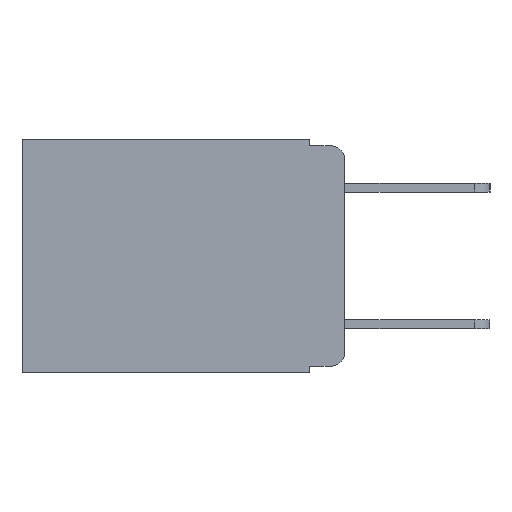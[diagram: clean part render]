
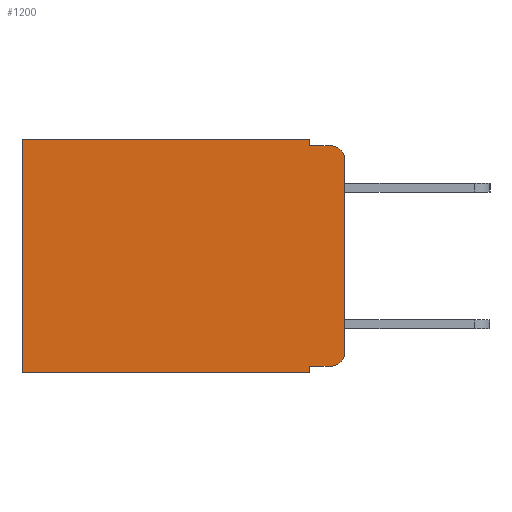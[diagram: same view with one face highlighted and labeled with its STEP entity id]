
A CAD part, left-side view. The second image highlights one B-rep face of the part: STEP entity #1200.
In plain terms, the highlighted planar face has unit normal (-1, 0, 0).
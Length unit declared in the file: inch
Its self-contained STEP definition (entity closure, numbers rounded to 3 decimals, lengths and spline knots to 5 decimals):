
#104 = DIRECTION ( 'NONE',  ( 0., 0., -1. ) ) ;
#127 = DIRECTION ( 'NONE',  ( -1., 0., 0. ) ) ;
#390 = LINE ( 'NONE', #4589, #6606 ) ;
#402 = DIRECTION ( 'NONE',  ( 1., 0., 0. ) ) ;
#555 = ORIENTED_EDGE ( 'NONE', *, *, #3717, .F. ) ;
#615 = VECTOR ( 'NONE', #10559, 39.37008 ) ;
#712 = VERTEX_POINT ( 'NONE', #10216 ) ;
#1023 = ORIENTED_EDGE ( 'NONE', *, *, #2513, .T. ) ;
#1200 = ADVANCED_FACE ( 'NONE', ( #3035 ), #11545, .F. ) ;
#1435 = ORIENTED_EDGE ( 'NONE', *, *, #3086, .F. ) ;
#1583 = CARTESIAN_POINT ( 'NONE',  ( 0.298, 0.02, -0.03 ) ) ;
#2192 = EDGE_CURVE ( 'NONE', #712, #9393, #390, .T. ) ;
#2199 = ORIENTED_EDGE ( 'NONE', *, *, #2450, .F. ) ;
#2424 = EDGE_CURVE ( 'NONE', #5941, #10983, #8377, .T. ) ;
#2448 = EDGE_CURVE ( 'NONE', #5403, #5941, #5868, .T. ) ;
#2450 = EDGE_CURVE ( 'NONE', #5403, #6132, #5561, .T. ) ;
#2513 = EDGE_CURVE ( 'NONE', #9393, #5995, #11016, .T. ) ;
#2515 = CARTESIAN_POINT ( 'NONE',  ( 0.298, 0.051, -0.333 ) ) ;
#2554 = AXIS2_PLACEMENT_3D ( 'NONE', #7008, #8761, #6050 ) ;
#2683 = ORIENTED_EDGE ( 'NONE', *, *, #3149, .F. ) ;
#2730 = DIRECTION ( 'NONE',  ( 0., 0., -1. ) ) ;
#3035 = FACE_OUTER_BOUND ( 'NONE', #11235, .T. ) ;
#3086 = EDGE_CURVE ( 'NONE', #712, #10606, #11137, .T. ) ;
#3087 = CARTESIAN_POINT ( 'NONE',  ( 0.298, 0.473, 0. ) ) ;
#3117 = AXIS2_PLACEMENT_3D ( 'NONE', #11617, #402, #11785 ) ;
#3149 = EDGE_CURVE ( 'NONE', #10606, #6322, #7765, .T. ) ;
#3220 = EDGE_CURVE ( 'NONE', #8643, #6322, #11270, .T. ) ;
#3293 = EDGE_CURVE ( 'NONE', #8643, #10983, #11638, .T. ) ;
#3717 = EDGE_CURVE ( 'NONE', #6132, #5995, #7465, .T. ) ;
#3788 = ORIENTED_EDGE ( 'NONE', *, *, #2424, .T. ) ;
#4033 = CARTESIAN_POINT ( 'NONE',  ( 0.298, 0.051, -0.01 ) ) ;
#4255 = CARTESIAN_POINT ( 'NONE',  ( 0.298, 0.473, -0.343 ) ) ;
#4398 = AXIS2_PLACEMENT_3D ( 'NONE', #1583, #127, #104 ) ;
#4589 = CARTESIAN_POINT ( 'NONE',  ( 0.298, 0., 0. ) ) ;
#4765 = DIRECTION ( 'NONE',  ( 0., 1., 0. ) ) ;
#4959 = CARTESIAN_POINT ( 'NONE',  ( 0.298, 0.051, -0.333 ) ) ;
#5037 = VECTOR ( 'NONE', #2730, 39.37008 ) ;
#5106 = DIRECTION ( 'NONE',  ( 0., 0., -1. ) ) ;
#5403 = VERTEX_POINT ( 'NONE', #2515 ) ;
#5487 = VECTOR ( 'NONE', #8368, 39.37008 ) ;
#5528 = ORIENTED_EDGE ( 'NONE', *, *, #2448, .T. ) ;
#5561 = LINE ( 'NONE', #10357, #7805 ) ;
#5868 = LINE ( 'NONE', #4959, #8072 ) ;
#5896 = DIRECTION ( 'NONE',  ( 0., -1., 0. ) ) ;
#5941 = VERTEX_POINT ( 'NONE', #6340 ) ;
#5995 = VERTEX_POINT ( 'NONE', #4255 ) ;
#6050 = DIRECTION ( 'NONE',  ( 0., 0., -1. ) ) ;
#6090 = DIRECTION ( 'NONE',  ( 0., -1., 0. ) ) ;
#6132 = VERTEX_POINT ( 'NONE', #9262 ) ;
#6187 = CARTESIAN_POINT ( 'NONE',  ( 0.298, 0.473, 0. ) ) ;
#6322 = VERTEX_POINT ( 'NONE', #11964 ) ;
#6340 = CARTESIAN_POINT ( 'NONE',  ( 0.298, 0.02, -0.333 ) ) ;
#6606 = VECTOR ( 'NONE', #4765, 39.37008 ) ;
#6925 = ORIENTED_EDGE ( 'NONE', *, *, #2192, .T. ) ;
#7008 = CARTESIAN_POINT ( 'NONE',  ( 0.298, 0.02, -0.313 ) ) ;
#7465 = LINE ( 'NONE', #10080, #5487 ) ;
#7765 = LINE ( 'NONE', #4033, #10336 ) ;
#7805 = VECTOR ( 'NONE', #5106, 39.37008 ) ;
#8072 = VECTOR ( 'NONE', #5896, 39.37008 ) ;
#8354 = DIRECTION ( 'NONE',  ( 0., 0., -1. ) ) ;
#8368 = DIRECTION ( 'NONE',  ( 0., 1., 0. ) ) ;
#8377 = CIRCLE ( 'NONE', #2554, 0.02 ) ;
#8643 = VERTEX_POINT ( 'NONE', #10036 ) ;
#8737 = ORIENTED_EDGE ( 'NONE', *, *, #3220, .T. ) ;
#8761 = DIRECTION ( 'NONE',  ( -1., 0., 0. ) ) ;
#9050 = CARTESIAN_POINT ( 'NONE',  ( 0.298, 0.051, -0.01 ) ) ;
#9262 = CARTESIAN_POINT ( 'NONE',  ( 0.298, 0.051, -0.343 ) ) ;
#9380 = CARTESIAN_POINT ( 'NONE',  ( 0.298, 0., -0.313 ) ) ;
#9393 = VERTEX_POINT ( 'NONE', #6187 ) ;
#10036 = CARTESIAN_POINT ( 'NONE',  ( 0.298, 0., -0.03 ) ) ;
#10045 = CARTESIAN_POINT ( 'NONE',  ( 0.298, 0.051, 0. ) ) ;
#10080 = CARTESIAN_POINT ( 'NONE',  ( 0.298, 0., -0.343 ) ) ;
#10216 = CARTESIAN_POINT ( 'NONE',  ( 0.298, 0.051, 0. ) ) ;
#10336 = VECTOR ( 'NONE', #6090, 39.37008 ) ;
#10357 = CARTESIAN_POINT ( 'NONE',  ( 0.298, 0.051, 0. ) ) ;
#10559 = DIRECTION ( 'NONE',  ( 0., 0., -1. ) ) ;
#10573 = CARTESIAN_POINT ( 'NONE',  ( 0.298, 0., 0. ) ) ;
#10606 = VERTEX_POINT ( 'NONE', #9050 ) ;
#10731 = VECTOR ( 'NONE', #8354, 39.37008 ) ;
#10983 = VERTEX_POINT ( 'NONE', #9380 ) ;
#11016 = LINE ( 'NONE', #3087, #10731 ) ;
#11137 = LINE ( 'NONE', #10045, #615 ) ;
#11235 = EDGE_LOOP ( 'NONE', ( #12009, #8737, #2683, #1435, #6925, #1023, #555, #2199, #5528, #3788 ) ) ;
#11270 = CIRCLE ( 'NONE', #4398, 0.02 ) ;
#11545 = PLANE ( 'NONE',  #3117 ) ;
#11617 = CARTESIAN_POINT ( 'NONE',  ( 0.298, 0., 0. ) ) ;
#11638 = LINE ( 'NONE', #10573, #5037 ) ;
#11785 = DIRECTION ( 'NONE',  ( 0., 0., -1. ) ) ;
#11964 = CARTESIAN_POINT ( 'NONE',  ( 0.298, 0.02, -0.01 ) ) ;
#12009 = ORIENTED_EDGE ( 'NONE', *, *, #3293, .F. ) ;
